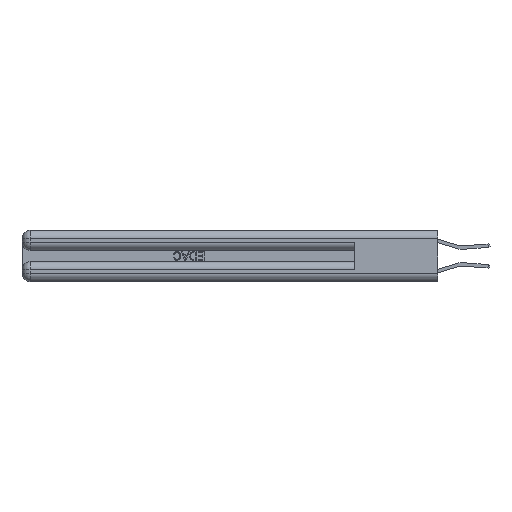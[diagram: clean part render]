
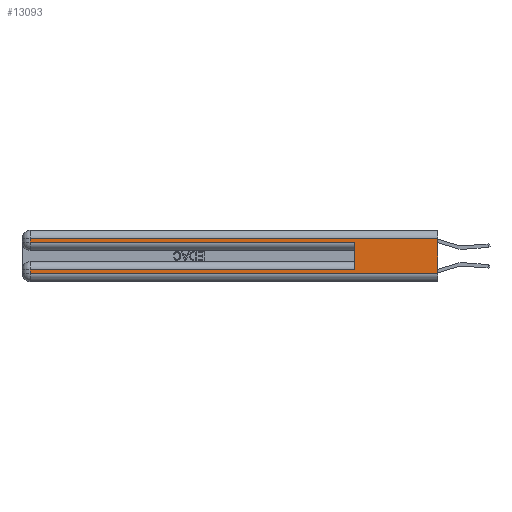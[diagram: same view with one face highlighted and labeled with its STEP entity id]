
A CAD part, left-side view. The second image highlights one B-rep face of the part: STEP entity #13093.
In plain terms, the highlighted planar face has unit normal (-1, 0, 0).
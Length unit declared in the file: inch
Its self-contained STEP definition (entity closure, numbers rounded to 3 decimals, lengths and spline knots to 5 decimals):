
#316 = VERTEX_POINT ( 'NONE', #20127 ) ;
#379 = VERTEX_POINT ( 'NONE', #10630 ) ;
#774 = EDGE_CURVE ( 'NONE', #316, #20579, #29077, .T. ) ;
#1012 = VECTOR ( 'NONE', #12297, 39.37008 ) ;
#1053 = VECTOR ( 'NONE', #18232, 39.37008 ) ;
#1265 = VERTEX_POINT ( 'NONE', #27454 ) ;
#1281 = FACE_OUTER_BOUND ( 'NONE', #5078, .T. ) ;
#1654 = VECTOR ( 'NONE', #16478, 39.37008 ) ;
#2272 = ORIENTED_EDGE ( 'NONE', *, *, #13907, .T. ) ;
#2482 = VERTEX_POINT ( 'NONE', #12659 ) ;
#2575 = DIRECTION ( 'NONE',  ( 0., 0., -1. ) ) ;
#3085 = LINE ( 'NONE', #9726, #1654 ) ;
#3493 = LINE ( 'NONE', #6553, #28282 ) ;
#3830 = ORIENTED_EDGE ( 'NONE', *, *, #20658, .F. ) ;
#5078 = EDGE_LOOP ( 'NONE', ( #3830, #2272, #7631, #21329, #20335, #28821, #8897, #11643 ) ) ;
#6553 = CARTESIAN_POINT ( 'NONE',  ( 0., 0., 0.37 ) ) ;
#7631 = ORIENTED_EDGE ( 'NONE', *, *, #774, .T. ) ;
#7829 = CARTESIAN_POINT ( 'NONE',  ( 0., 0.6, 0.145 ) ) ;
#8897 = ORIENTED_EDGE ( 'NONE', *, *, #17118, .T. ) ;
#9726 = CARTESIAN_POINT ( 'NONE',  ( 0., 2.94, 0.37 ) ) ;
#9794 = CARTESIAN_POINT ( 'NONE',  ( 0., 0., 0.31 ) ) ;
#9843 = LINE ( 'NONE', #28087, #25847 ) ;
#10092 = CARTESIAN_POINT ( 'NONE',  ( 0., 2.94, 0.06 ) ) ;
#10630 = CARTESIAN_POINT ( 'NONE',  ( 0., 2.94, 0.085 ) ) ;
#11187 = DIRECTION ( 'NONE',  ( 0., 0., -1. ) ) ;
#11643 = ORIENTED_EDGE ( 'NONE', *, *, #13368, .T. ) ;
#11752 = DIRECTION ( 'NONE',  ( 0., 1., 0. ) ) ;
#12027 = CARTESIAN_POINT ( 'NONE',  ( 0., 0., 0.31 ) ) ;
#12297 = DIRECTION ( 'NONE',  ( 0., 0., 1. ) ) ;
#12659 = CARTESIAN_POINT ( 'NONE',  ( 0., 0., 0.06 ) ) ;
#13093 = ADVANCED_FACE ( 'NONE', ( #1281 ), #14024, .F. ) ;
#13368 = EDGE_CURVE ( 'NONE', #18608, #2482, #23795, .T. ) ;
#13377 = CARTESIAN_POINT ( 'NONE',  ( 0., 2.94, 0.37 ) ) ;
#13907 = EDGE_CURVE ( 'NONE', #26485, #316, #16094, .T. ) ;
#14018 = VERTEX_POINT ( 'NONE', #26395 ) ;
#14024 = PLANE ( 'NONE',  #29672 ) ;
#14518 = CARTESIAN_POINT ( 'NONE',  ( 0., 0., 0.06 ) ) ;
#16094 = LINE ( 'NONE', #12027, #23732 ) ;
#16478 = DIRECTION ( 'NONE',  ( 0., 0., -1. ) ) ;
#17118 = EDGE_CURVE ( 'NONE', #379, #18608, #3085, .T. ) ;
#17160 = DIRECTION ( 'NONE',  ( 0., -1., 0. ) ) ;
#17819 = CARTESIAN_POINT ( 'NONE',  ( 0., 2.94, 0.285 ) ) ;
#18232 = DIRECTION ( 'NONE',  ( 0., 0., -1. ) ) ;
#18608 = VERTEX_POINT ( 'NONE', #10092 ) ;
#19276 = LINE ( 'NONE', #7829, #1012 ) ;
#19716 = EDGE_CURVE ( 'NONE', #14018, #1265, #19276, .T. ) ;
#20127 = CARTESIAN_POINT ( 'NONE',  ( 0., 2.94, 0.31 ) ) ;
#20335 = ORIENTED_EDGE ( 'NONE', *, *, #19716, .F. ) ;
#20579 = VERTEX_POINT ( 'NONE', #17819 ) ;
#20658 = EDGE_CURVE ( 'NONE', #26485, #2482, #3493, .T. ) ;
#20888 = VECTOR ( 'NONE', #17160, 39.37008 ) ;
#21117 = DIRECTION ( 'NONE',  ( 1., 0., 0. ) ) ;
#21329 = ORIENTED_EDGE ( 'NONE', *, *, #26140, .T. ) ;
#23459 = CARTESIAN_POINT ( 'NONE',  ( 0., 0., 0.37 ) ) ;
#23732 = VECTOR ( 'NONE', #28251, 39.37008 ) ;
#23795 = LINE ( 'NONE', #14518, #20888 ) ;
#24000 = VECTOR ( 'NONE', #24379, 39.37008 ) ;
#24379 = DIRECTION ( 'NONE',  ( 0., -1., 0. ) ) ;
#24776 = CARTESIAN_POINT ( 'NONE',  ( 0., 0., 0.285 ) ) ;
#25847 = VECTOR ( 'NONE', #11752, 39.37008 ) ;
#26140 = EDGE_CURVE ( 'NONE', #20579, #1265, #27997, .T. ) ;
#26395 = CARTESIAN_POINT ( 'NONE',  ( 0., 0.6, 0.085 ) ) ;
#26485 = VERTEX_POINT ( 'NONE', #9794 ) ;
#27135 = EDGE_CURVE ( 'NONE', #14018, #379, #9843, .T. ) ;
#27454 = CARTESIAN_POINT ( 'NONE',  ( 0., 0.6, 0.285 ) ) ;
#27997 = LINE ( 'NONE', #24776, #24000 ) ;
#28087 = CARTESIAN_POINT ( 'NONE',  ( 0., 0., 0.085 ) ) ;
#28251 = DIRECTION ( 'NONE',  ( 0., 1., 0. ) ) ;
#28282 = VECTOR ( 'NONE', #11187, 39.37008 ) ;
#28821 = ORIENTED_EDGE ( 'NONE', *, *, #27135, .T. ) ;
#29077 = LINE ( 'NONE', #13377, #1053 ) ;
#29672 = AXIS2_PLACEMENT_3D ( 'NONE', #23459, #21117, #2575 ) ;
